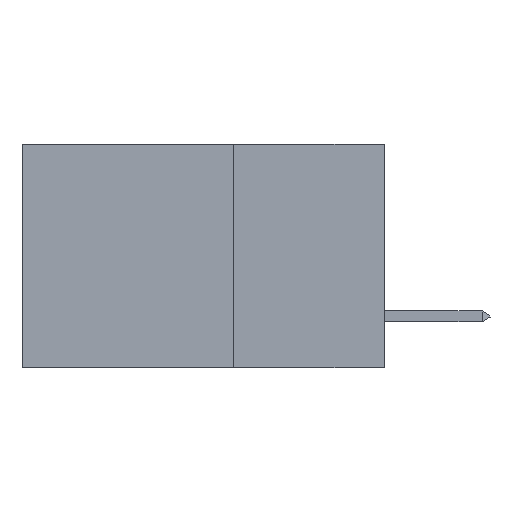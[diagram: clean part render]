
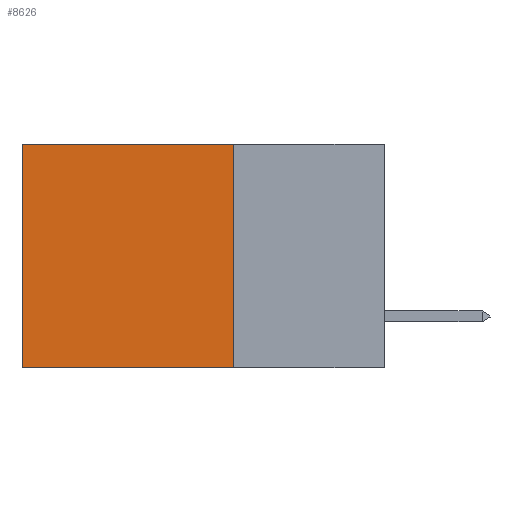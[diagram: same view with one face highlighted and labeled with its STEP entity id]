
A CAD part, left-side view. The second image highlights one B-rep face of the part: STEP entity #8626.
In plain terms, the highlighted planar face has unit normal (-1, 0, 0).
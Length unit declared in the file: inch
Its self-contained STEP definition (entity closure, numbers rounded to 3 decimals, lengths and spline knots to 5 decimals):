
#166 = DIRECTION ( 'NONE',  ( 1., 0., 0. ) ) ;
#273 = VERTEX_POINT ( 'NONE', #4630 ) ;
#629 = CARTESIAN_POINT ( 'NONE',  ( 0.2875, 0.25, -0.37 ) ) ;
#1208 = AXIS2_PLACEMENT_3D ( 'NONE', #6599, #166, #7580 ) ;
#1237 = ORIENTED_EDGE ( 'NONE', *, *, #2957, .T. ) ;
#1973 = DIRECTION ( 'NONE',  ( 0., 0., -1. ) ) ;
#2165 = VERTEX_POINT ( 'NONE', #629 ) ;
#2498 = EDGE_CURVE ( 'NONE', #5897, #273, #5761, .T. ) ;
#2665 = FACE_OUTER_BOUND ( 'NONE', #3555, .T. ) ;
#2957 = EDGE_CURVE ( 'NONE', #6556, #5897, #3679, .T. ) ;
#2959 = PLANE ( 'NONE',  #1208 ) ;
#3370 = ORIENTED_EDGE ( 'NONE', *, *, #10720, .F. ) ;
#3555 = EDGE_LOOP ( 'NONE', ( #10191, #8991, #3370, #1237 ) ) ;
#3679 = LINE ( 'NONE', #4469, #8459 ) ;
#3996 = VECTOR ( 'NONE', #1973, 39.37008 ) ;
#4469 = CARTESIAN_POINT ( 'NONE',  ( 0.2875, 0.25, 0. ) ) ;
#4511 = DIRECTION ( 'NONE',  ( 0., 1., 0. ) ) ;
#4630 = CARTESIAN_POINT ( 'NONE',  ( 0.2875, 0.6, -0.37 ) ) ;
#4959 = CARTESIAN_POINT ( 'NONE',  ( 0.2875, 0.25, -0.37 ) ) ;
#5088 = LINE ( 'NONE', #6147, #7557 ) ;
#5761 = LINE ( 'NONE', #7478, #3996 ) ;
#5897 = VERTEX_POINT ( 'NONE', #6191 ) ;
#6147 = CARTESIAN_POINT ( 'NONE',  ( 0.2875, 0.25, 0. ) ) ;
#6191 = CARTESIAN_POINT ( 'NONE',  ( 0.2875, 0.6, 0. ) ) ;
#6556 = VERTEX_POINT ( 'NONE', #8961 ) ;
#6599 = CARTESIAN_POINT ( 'NONE',  ( 0.2875, 0.25, 0. ) ) ;
#7478 = CARTESIAN_POINT ( 'NONE',  ( 0.2875, 0.6, 0. ) ) ;
#7557 = VECTOR ( 'NONE', #9874, 39.37008 ) ;
#7580 = DIRECTION ( 'NONE',  ( 0., 0., -1. ) ) ;
#7997 = EDGE_CURVE ( 'NONE', #2165, #273, #8040, .T. ) ;
#8040 = LINE ( 'NONE', #4959, #10081 ) ;
#8459 = VECTOR ( 'NONE', #4511, 39.37008 ) ;
#8626 = ADVANCED_FACE ( 'NONE', ( #2665 ), #2959, .F. ) ;
#8961 = CARTESIAN_POINT ( 'NONE',  ( 0.2875, 0.25, 0. ) ) ;
#8991 = ORIENTED_EDGE ( 'NONE', *, *, #7997, .F. ) ;
#9523 = DIRECTION ( 'NONE',  ( 0., 1., 0. ) ) ;
#9874 = DIRECTION ( 'NONE',  ( 0., 0., -1. ) ) ;
#10081 = VECTOR ( 'NONE', #9523, 39.37008 ) ;
#10191 = ORIENTED_EDGE ( 'NONE', *, *, #2498, .T. ) ;
#10720 = EDGE_CURVE ( 'NONE', #6556, #2165, #5088, .T. ) ;
